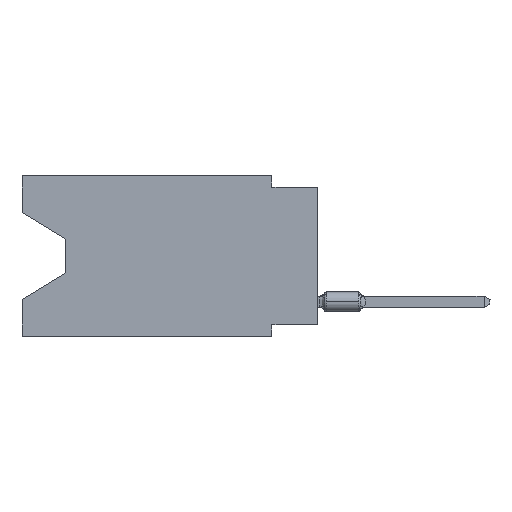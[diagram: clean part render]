
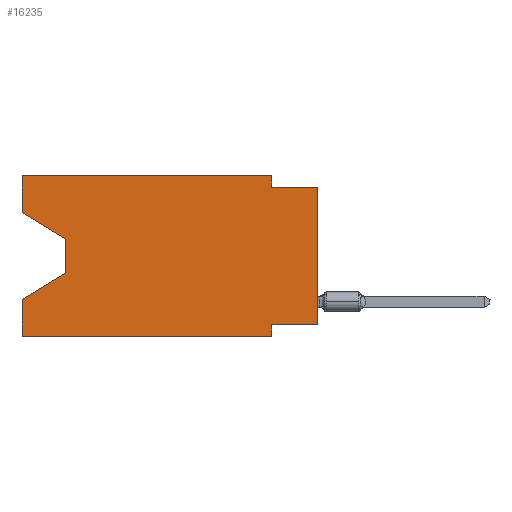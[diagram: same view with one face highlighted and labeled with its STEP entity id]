
A CAD part, left-side view. The second image highlights one B-rep face of the part: STEP entity #16235.
In plain terms, the highlighted planar face has unit normal (-1, 0, 0).
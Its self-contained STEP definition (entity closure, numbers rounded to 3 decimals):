
#149 = LINE ( 'NONE', #15773, #14087 ) ;
#286 = EDGE_CURVE ( 'NONE', #37078, #23345, #28996, .T. ) ;
#353 = CARTESIAN_POINT ( 'NONE',  ( 0., 0., -8.255 ) ) ;
#393 = VERTEX_POINT ( 'NONE', #59515 ) ;
#746 = EDGE_CURVE ( 'NONE', #37078, #28251, #27342, .T. ) ;
#929 = VECTOR ( 'NONE', #23491, 1000. ) ;
#1416 = AXIS2_PLACEMENT_3D ( 'NONE', #9489, #40052, #59736 ) ;
#5326 = ORIENTED_EDGE ( 'NONE', *, *, #77427, .T. ) ;
#6493 = CARTESIAN_POINT ( 'NONE',  ( 0., 0., -0.635 ) ) ;
#6827 = DIRECTION ( 'NONE',  ( 0., 0., -1. ) ) ;
#6933 = ORIENTED_EDGE ( 'NONE', *, *, #65544, .F. ) ;
#8413 = VECTOR ( 'NONE', #37850, 1000. ) ;
#9011 = ORIENTED_EDGE ( 'NONE', *, *, #67078, .F. ) ;
#9489 = CARTESIAN_POINT ( 'NONE',  ( 0., 16.383, 0. ) ) ;
#10779 = CARTESIAN_POINT ( 'NONE',  ( 0., 0., -8.255 ) ) ;
#11121 = VECTOR ( 'NONE', #6827, 1000. ) ;
#11369 = EDGE_CURVE ( 'NONE', #12134, #15128, #29859, .T. ) ;
#11623 = CARTESIAN_POINT ( 'NONE',  ( 0., 16.383, 0. ) ) ;
#12134 = VERTEX_POINT ( 'NONE', #35630 ) ;
#12632 = DIRECTION ( 'NONE',  ( 0., 1., 0. ) ) ;
#12780 = ORIENTED_EDGE ( 'NONE', *, *, #286, .T. ) ;
#12788 = LINE ( 'NONE', #11623, #32937 ) ;
#14087 = VECTOR ( 'NONE', #78318, 1000. ) ;
#14579 = CARTESIAN_POINT ( 'NONE',  ( 0., 13.97, -5.385 ) ) ;
#15128 = VERTEX_POINT ( 'NONE', #48990 ) ;
#15448 = PLANE ( 'NONE',  #1416 ) ;
#15773 = CARTESIAN_POINT ( 'NONE',  ( 0., 2.54, -8.89 ) ) ;
#16235 = ADVANCED_FACE ( 'NONE', ( #21015 ), #15448, .F. ) ;
#16753 = EDGE_CURVE ( 'NONE', #393, #23345, #149, .T. ) ;
#19688 = EDGE_LOOP ( 'NONE', ( #47198, #5326, #67930, #24166, #12780, #43302, #56088, #73067, #6933, #31006, #9011, #49761 ) ) ;
#21015 = FACE_OUTER_BOUND ( 'NONE', #19688, .T. ) ;
#21483 = CARTESIAN_POINT ( 'NONE',  ( 0., 16.383, -8.89 ) ) ;
#22397 = EDGE_CURVE ( 'NONE', #71046, #77077, #22730, .T. ) ;
#22481 = LINE ( 'NONE', #71250, #51744 ) ;
#22730 = LINE ( 'NONE', #48058, #28974 ) ;
#23345 = VERTEX_POINT ( 'NONE', #37427 ) ;
#23491 = DIRECTION ( 'NONE',  ( 0., -0.855, -0.519 ) ) ;
#24166 = ORIENTED_EDGE ( 'NONE', *, *, #746, .F. ) ;
#25135 = DIRECTION ( 'NONE',  ( 0., -1., 0. ) ) ;
#25163 = LINE ( 'NONE', #69175, #8413 ) ;
#25911 = LINE ( 'NONE', #6493, #64444 ) ;
#26072 = VECTOR ( 'NONE', #75869, 1000. ) ;
#27342 = LINE ( 'NONE', #51536, #66841 ) ;
#28251 = VERTEX_POINT ( 'NONE', #78344 ) ;
#28974 = VECTOR ( 'NONE', #42122, 1000. ) ;
#28996 = LINE ( 'NONE', #21483, #62877 ) ;
#29859 = LINE ( 'NONE', #54052, #11121 ) ;
#30700 = VERTEX_POINT ( 'NONE', #42916 ) ;
#31006 = ORIENTED_EDGE ( 'NONE', *, *, #11369, .F. ) ;
#31524 = EDGE_CURVE ( 'NONE', #72114, #28251, #25163, .T. ) ;
#32937 = VECTOR ( 'NONE', #67560, 1000. ) ;
#34754 = DIRECTION ( 'NONE',  ( 0., 0., -1. ) ) ;
#35630 = CARTESIAN_POINT ( 'NONE',  ( 0., 2.54, 0. ) ) ;
#37078 = VERTEX_POINT ( 'NONE', #49997 ) ;
#37239 = LINE ( 'NONE', #353, #67685 ) ;
#37427 = CARTESIAN_POINT ( 'NONE',  ( 0., 2.54, -8.89 ) ) ;
#37850 = DIRECTION ( 'NONE',  ( 0., 0.855, -0.519 ) ) ;
#40052 = DIRECTION ( 'NONE',  ( 1., 0., 0. ) ) ;
#41194 = CARTESIAN_POINT ( 'NONE',  ( 0., 0., -0.635 ) ) ;
#42122 = DIRECTION ( 'NONE',  ( 0., 0., 1. ) ) ;
#42511 = LINE ( 'NONE', #65542, #929 ) ;
#42916 = CARTESIAN_POINT ( 'NONE',  ( 0., 16.383, -2.038 ) ) ;
#43302 = ORIENTED_EDGE ( 'NONE', *, *, #16753, .F. ) ;
#44234 = EDGE_CURVE ( 'NONE', #30700, #55535, #42511, .T. ) ;
#46501 = CARTESIAN_POINT ( 'NONE',  ( 0., 16.383, 0. ) ) ;
#47198 = ORIENTED_EDGE ( 'NONE', *, *, #44234, .T. ) ;
#48058 = CARTESIAN_POINT ( 'NONE',  ( 0., 0., 0. ) ) ;
#48990 = CARTESIAN_POINT ( 'NONE',  ( 0., 2.54, -0.635 ) ) ;
#49761 = ORIENTED_EDGE ( 'NONE', *, *, #50444, .F. ) ;
#49997 = CARTESIAN_POINT ( 'NONE',  ( 0., 16.383, -8.89 ) ) ;
#50444 = EDGE_CURVE ( 'NONE', #30700, #61749, #70711, .T. ) ;
#51536 = CARTESIAN_POINT ( 'NONE',  ( 0., 16.383, 0. ) ) ;
#51744 = VECTOR ( 'NONE', #34754, 1000. ) ;
#53698 = CARTESIAN_POINT ( 'NONE',  ( 0., 16.383, 0. ) ) ;
#54000 = CARTESIAN_POINT ( 'NONE',  ( 0., 13.97, -3.505 ) ) ;
#54052 = CARTESIAN_POINT ( 'NONE',  ( 0., 2.54, 0. ) ) ;
#55535 = VERTEX_POINT ( 'NONE', #54000 ) ;
#56088 = ORIENTED_EDGE ( 'NONE', *, *, #73245, .F. ) ;
#59515 = CARTESIAN_POINT ( 'NONE',  ( 0., 2.54, -8.255 ) ) ;
#59736 = DIRECTION ( 'NONE',  ( 0., 0., -1. ) ) ;
#61749 = VERTEX_POINT ( 'NONE', #53698 ) ;
#62877 = VECTOR ( 'NONE', #76229, 1000. ) ;
#64444 = VECTOR ( 'NONE', #25135, 1000. ) ;
#65542 = CARTESIAN_POINT ( 'NONE',  ( 0., 16.383, -2.038 ) ) ;
#65544 = EDGE_CURVE ( 'NONE', #15128, #77077, #25911, .T. ) ;
#66841 = VECTOR ( 'NONE', #75750, 1000. ) ;
#67078 = EDGE_CURVE ( 'NONE', #61749, #12134, #12788, .T. ) ;
#67560 = DIRECTION ( 'NONE',  ( 0., -1., 0. ) ) ;
#67685 = VECTOR ( 'NONE', #12632, 1000. ) ;
#67930 = ORIENTED_EDGE ( 'NONE', *, *, #31524, .T. ) ;
#69175 = CARTESIAN_POINT ( 'NONE',  ( 0., 13.97, -5.385 ) ) ;
#70711 = LINE ( 'NONE', #46501, #26072 ) ;
#71046 = VERTEX_POINT ( 'NONE', #10779 ) ;
#71250 = CARTESIAN_POINT ( 'NONE',  ( 0., 13.97, -3.505 ) ) ;
#72114 = VERTEX_POINT ( 'NONE', #14579 ) ;
#73067 = ORIENTED_EDGE ( 'NONE', *, *, #22397, .T. ) ;
#73245 = EDGE_CURVE ( 'NONE', #71046, #393, #37239, .T. ) ;
#75750 = DIRECTION ( 'NONE',  ( 0., 0., 1. ) ) ;
#75869 = DIRECTION ( 'NONE',  ( 0., 0., 1. ) ) ;
#76229 = DIRECTION ( 'NONE',  ( 0., -1., 0. ) ) ;
#77077 = VERTEX_POINT ( 'NONE', #41194 ) ;
#77427 = EDGE_CURVE ( 'NONE', #55535, #72114, #22481, .T. ) ;
#78318 = DIRECTION ( 'NONE',  ( 0., 0., -1. ) ) ;
#78344 = CARTESIAN_POINT ( 'NONE',  ( 0., 16.383, -6.852 ) ) ;
